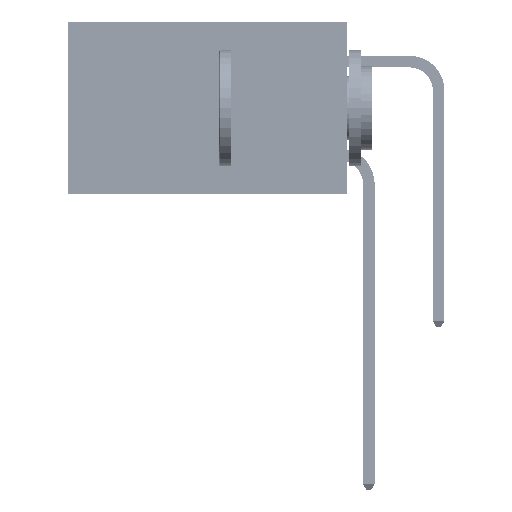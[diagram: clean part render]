
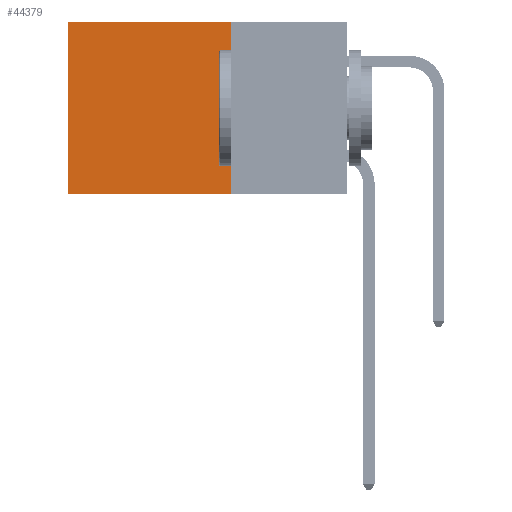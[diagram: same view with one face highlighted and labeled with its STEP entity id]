
A CAD part, left-side view. The second image highlights one B-rep face of the part: STEP entity #44379.
In plain terms, the highlighted planar face has unit normal (-1, 0, 0).
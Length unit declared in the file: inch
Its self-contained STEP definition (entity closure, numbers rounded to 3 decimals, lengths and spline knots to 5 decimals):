
#1234 = DIRECTION ( 'NONE',  ( 0., 1., 0. ) ) ;
#1915 = CARTESIAN_POINT ( 'NONE',  ( 0.2875, 0.25, 0. ) ) ;
#4727 = VECTOR ( 'NONE', #8574, 39.37008 ) ;
#8100 = CARTESIAN_POINT ( 'NONE',  ( 0.2875, 0.6, -0.37 ) ) ;
#8574 = DIRECTION ( 'NONE',  ( 0., 0., -1. ) ) ;
#10500 = VERTEX_POINT ( 'NONE', #8100 ) ;
#10591 = EDGE_LOOP ( 'NONE', ( #11849, #13292, #34235, #20197 ) ) ;
#11149 = CARTESIAN_POINT ( 'NONE',  ( 0.2875, 0.25, 0. ) ) ;
#11773 = VERTEX_POINT ( 'NONE', #1915 ) ;
#11849 = ORIENTED_EDGE ( 'NONE', *, *, #31813, .T. ) ;
#12257 = CARTESIAN_POINT ( 'NONE',  ( 0.2875, 0.6, 0. ) ) ;
#13292 = ORIENTED_EDGE ( 'NONE', *, *, #38366, .F. ) ;
#14952 = DIRECTION ( 'NONE',  ( 0., 0., -1. ) ) ;
#16453 = VECTOR ( 'NONE', #38190, 39.37008 ) ;
#17550 = EDGE_CURVE ( 'NONE', #11773, #34065, #41484, .T. ) ;
#19249 = LINE ( 'NONE', #38860, #39333 ) ;
#20197 = ORIENTED_EDGE ( 'NONE', *, *, #17550, .T. ) ;
#23820 = CARTESIAN_POINT ( 'NONE',  ( 0.2875, 0.25, -0.37 ) ) ;
#25133 = FACE_OUTER_BOUND ( 'NONE', #10591, .T. ) ;
#26729 = VECTOR ( 'NONE', #1234, 39.37008 ) ;
#31183 = CARTESIAN_POINT ( 'NONE',  ( 0.2875, 0.25, 0. ) ) ;
#31813 = EDGE_CURVE ( 'NONE', #34065, #10500, #48467, .T. ) ;
#33496 = PLANE ( 'NONE',  #35433 ) ;
#34065 = VERTEX_POINT ( 'NONE', #38525 ) ;
#34235 = ORIENTED_EDGE ( 'NONE', *, *, #43490, .F. ) ;
#35433 = AXIS2_PLACEMENT_3D ( 'NONE', #11149, #37617, #14952 ) ;
#37617 = DIRECTION ( 'NONE',  ( 1., 0., 0. ) ) ;
#38190 = DIRECTION ( 'NONE',  ( 0., 1., 0. ) ) ;
#38366 = EDGE_CURVE ( 'NONE', #45382, #10500, #46573, .T. ) ;
#38525 = CARTESIAN_POINT ( 'NONE',  ( 0.2875, 0.6, 0. ) ) ;
#38860 = CARTESIAN_POINT ( 'NONE',  ( 0.2875, 0.25, 0. ) ) ;
#39333 = VECTOR ( 'NONE', #46422, 39.37008 ) ;
#41484 = LINE ( 'NONE', #31183, #26729 ) ;
#43490 = EDGE_CURVE ( 'NONE', #11773, #45382, #19249, .T. ) ;
#44379 = ADVANCED_FACE ( 'NONE', ( #25133 ), #33496, .F. ) ;
#45382 = VERTEX_POINT ( 'NONE', #23820 ) ;
#45902 = CARTESIAN_POINT ( 'NONE',  ( 0.2875, 0.25, -0.37 ) ) ;
#46422 = DIRECTION ( 'NONE',  ( 0., 0., -1. ) ) ;
#46573 = LINE ( 'NONE', #45902, #16453 ) ;
#48467 = LINE ( 'NONE', #12257, #4727 ) ;
